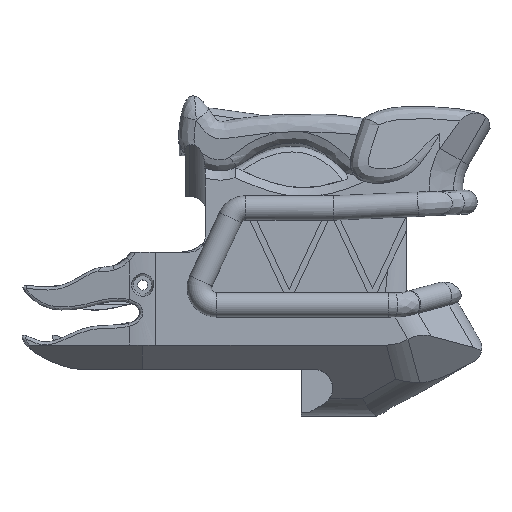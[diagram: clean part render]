
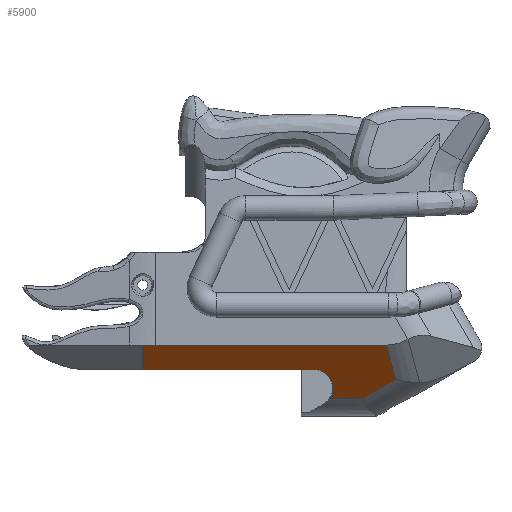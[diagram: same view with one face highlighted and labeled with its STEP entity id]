
A CAD part, left-side view. The second image highlights one B-rep face of the part: STEP entity #5900.
In plain terms, the highlighted planar face has unit normal (-0.707, 0, -0.707).
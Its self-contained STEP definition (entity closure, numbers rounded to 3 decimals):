
#164=PLANE('',#6316);
#215=LINE('',#8056,#571);
#218=LINE('',#8095,#574);
#220=LINE('',#8101,#576);
#506=LINE('',#30148,#862);
#508=LINE('',#30155,#864);
#511=LINE('',#30160,#867);
#514=LINE('',#30167,#870);
#571=VECTOR('',#6479,10.);
#574=VECTOR('',#6490,10.);
#576=VECTOR('',#6496,10.);
#862=VECTOR('',#7424,10.);
#864=VECTOR('',#7432,10.);
#867=VECTOR('',#7437,10.);
#870=VECTOR('',#7446,10.);
#1586=FACE_OUTER_BOUND('',#1890,.T.);
#1890=EDGE_LOOP('',(#5494,#5495,#5496,#5497,#5498,#5499,#5500,#5501,#5502,
#5503));
#1923=ELLIPSE('',#5985,8.485,6.);
#1994=ELLIPSE('',#6299,8.485,6.);
#1995=ELLIPSE('',#6303,70.711,50.);
#2201=VERTEX_POINT('',#8053);
#2202=VERTEX_POINT('',#8055);
#2208=VERTEX_POINT('',#8093);
#2210=VERTEX_POINT('',#8099);
#2216=VERTEX_POINT('',#8120);
#2727=VERTEX_POINT('',#30146);
#2728=VERTEX_POINT('',#30150);
#2729=VERTEX_POINT('',#30154);
#2730=VERTEX_POINT('',#30158);
#2731=VERTEX_POINT('',#30162);
#2848=EDGE_CURVE('',#2201,#2202,#215,.T.);
#2856=EDGE_CURVE('',#2208,#2201,#218,.T.);
#2859=EDGE_CURVE('',#2210,#2208,#220,.T.);
#2869=EDGE_CURVE('',#2202,#2216,#1923,.T.);
#3637=EDGE_CURVE('',#2216,#2727,#506,.T.);
#3638=EDGE_CURVE('',#2727,#2728,#1994,.T.);
#3640=EDGE_CURVE('',#2728,#2729,#508,.T.);
#3643=EDGE_CURVE('',#2729,#2730,#511,.T.);
#3644=EDGE_CURVE('',#2730,#2731,#1995,.T.);
#3647=EDGE_CURVE('',#2210,#2731,#514,.T.);
#5494=ORIENTED_EDGE('',*,*,#2859,.F.);
#5495=ORIENTED_EDGE('',*,*,#3647,.T.);
#5496=ORIENTED_EDGE('',*,*,#3644,.F.);
#5497=ORIENTED_EDGE('',*,*,#3643,.F.);
#5498=ORIENTED_EDGE('',*,*,#3640,.F.);
#5499=ORIENTED_EDGE('',*,*,#3638,.F.);
#5500=ORIENTED_EDGE('',*,*,#3637,.F.);
#5501=ORIENTED_EDGE('',*,*,#2869,.F.);
#5502=ORIENTED_EDGE('',*,*,#2848,.F.);
#5503=ORIENTED_EDGE('',*,*,#2856,.F.);
#5900=ADVANCED_FACE('',(#1586),#164,.T.);
#5985=AXIS2_PLACEMENT_3D('',#8121,#6518,#6519);
#6299=AXIS2_PLACEMENT_3D('',#30151,#7427,#7428);
#6303=AXIS2_PLACEMENT_3D('',#30163,#7440,#7441);
#6316=AXIS2_PLACEMENT_3D('',#30186,#7476,#7477);
#6479=DIRECTION('',(0.,1.,0.));
#6490=DIRECTION('',(0.447,0.775,-0.447));
#6496=DIRECTION('',(0.695,-0.186,-0.695));
#6518=DIRECTION('center_axis',(-0.707,0.,
-0.707));
#6519=DIRECTION('ref_axis',(0.707,0.,-0.707));
#7424=DIRECTION('',(-0.695,0.186,0.695));
#7427=DIRECTION('center_axis',(-0.707,0.,
-0.707));
#7428=DIRECTION('ref_axis',(-0.707,0.,0.707));
#7432=DIRECTION('',(0.,1.,0.));
#7437=DIRECTION('',(-0.707,0.,0.707));
#7440=DIRECTION('center_axis',(0.707,0.,
0.707));
#7441=DIRECTION('ref_axis',(-0.707,0.,0.707));
#7446=DIRECTION('',(0.,1.,0.));
#7476=DIRECTION('center_axis',(-0.707,0.,
-0.707));
#7477=DIRECTION('ref_axis',(-0.707,0.,0.707));
#8053=CARTESIAN_POINT('',(-12.533,-35.001,-59.547));
#8055=CARTESIAN_POINT('',(-12.533,-24.223,-59.547));
#8056=CARTESIAN_POINT('',(-12.533,-37.906,-59.547));
#8093=CARTESIAN_POINT('',(-18.787,-45.834,-53.293));
#8095=CARTESIAN_POINT('',(-21.885,-51.2,-50.195));
#8099=CARTESIAN_POINT('',(-30.,-42.829,-42.08));
#8101=CARTESIAN_POINT('',(-22.253,-44.905,-49.827));
#8120=CARTESIAN_POINT('',(-17.376,-25.001,-54.704));
#8121=CARTESIAN_POINT('Origin',(-15.823,-19.205,-56.257));
#30146=CARTESIAN_POINT('',(-17.553,-24.954,-54.527));
#30148=CARTESIAN_POINT('',(-19.247,-24.5,-52.833));
#30150=CARTESIAN_POINT('',(-22.,-19.158,-50.08));
#30151=CARTESIAN_POINT('Origin',(-16.,-19.158,-56.08));
#30154=CARTESIAN_POINT('',(-22.,37.17,-50.08));
#30155=CARTESIAN_POINT('',(-22.,-18.971,-50.08));
#30158=CARTESIAN_POINT('',(-29.808,37.17,-42.272));
#30160=CARTESIAN_POINT('',(-31.492,37.17,-40.588));
#30162=CARTESIAN_POINT('',(-30.,32.796,-42.08));
#30163=CARTESIAN_POINT('Origin',(20.,32.796,-92.08));
#30167=CARTESIAN_POINT('',(-30.,-37.98,-42.08));
#30186=CARTESIAN_POINT('Origin',(-26.,-37.98,-46.08));
